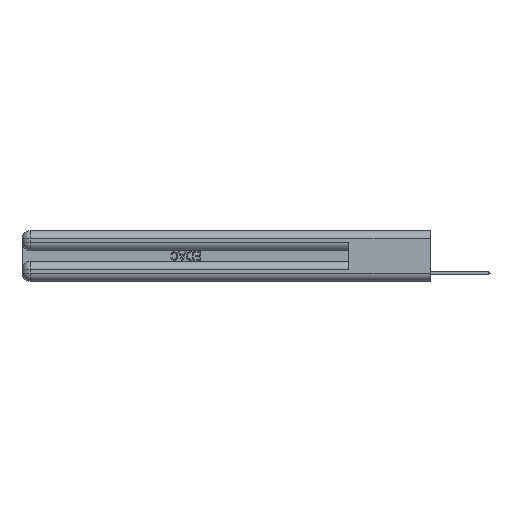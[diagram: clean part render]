
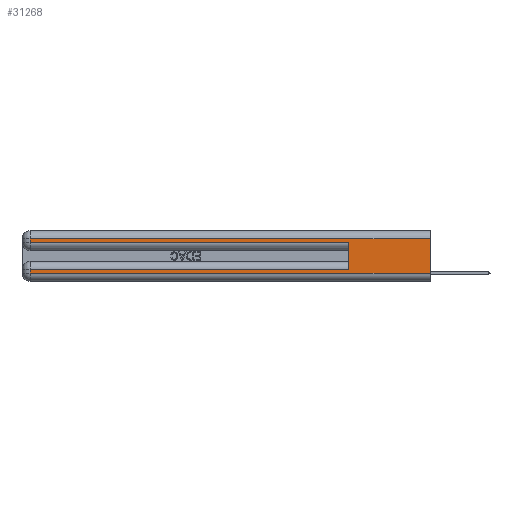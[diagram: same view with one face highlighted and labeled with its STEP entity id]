
A CAD part, left-side view. The second image highlights one B-rep face of the part: STEP entity #31268.
In plain terms, the highlighted planar face has unit normal (-1, 0, 0).
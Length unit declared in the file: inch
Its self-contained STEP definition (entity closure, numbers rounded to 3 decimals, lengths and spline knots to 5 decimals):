
#842 = DIRECTION ( 'NONE',  ( 0., 0., -1. ) ) ;
#1890 = LINE ( 'NONE', #7753, #27361 ) ;
#2162 = DIRECTION ( 'NONE',  ( 0., 0., -1. ) ) ;
#2788 = CARTESIAN_POINT ( 'NONE',  ( 0., 0., 0.085 ) ) ;
#2800 = VERTEX_POINT ( 'NONE', #10243 ) ;
#2830 = LINE ( 'NONE', #23119, #6940 ) ;
#3076 = VERTEX_POINT ( 'NONE', #11005 ) ;
#3846 = VERTEX_POINT ( 'NONE', #15947 ) ;
#3997 = CARTESIAN_POINT ( 'NONE',  ( 0., 2.94, 0.085 ) ) ;
#4005 = PLANE ( 'NONE',  #29487 ) ;
#4246 = VECTOR ( 'NONE', #32709, 39.37008 ) ;
#4670 = FACE_OUTER_BOUND ( 'NONE', #17009, .T. ) ;
#6491 = CARTESIAN_POINT ( 'NONE',  ( 0., 0.6, 0.145 ) ) ;
#6702 = VECTOR ( 'NONE', #842, 39.37008 ) ;
#6940 = VECTOR ( 'NONE', #13075, 39.37008 ) ;
#7240 = EDGE_CURVE ( 'NONE', #3846, #18724, #27258, .T. ) ;
#7455 = CARTESIAN_POINT ( 'NONE',  ( 0., 0., 0.37 ) ) ;
#7561 = LINE ( 'NONE', #21481, #6702 ) ;
#7753 = CARTESIAN_POINT ( 'NONE',  ( 0., 2.94, 0.37 ) ) ;
#7804 = DIRECTION ( 'NONE',  ( 0., 1., 0. ) ) ;
#8552 = EDGE_CURVE ( 'NONE', #9282, #28217, #1890, .T. ) ;
#9282 = VERTEX_POINT ( 'NONE', #3997 ) ;
#9346 = DIRECTION ( 'NONE',  ( 0., 0., 1. ) ) ;
#9461 = VERTEX_POINT ( 'NONE', #14901 ) ;
#10243 = CARTESIAN_POINT ( 'NONE',  ( 0., 0.6, 0.085 ) ) ;
#11005 = CARTESIAN_POINT ( 'NONE',  ( 0., 2.94, 0.285 ) ) ;
#11132 = EDGE_CURVE ( 'NONE', #2800, #9282, #13342, .T. ) ;
#12119 = ORIENTED_EDGE ( 'NONE', *, *, #7240, .F. ) ;
#12609 = LINE ( 'NONE', #17635, #4246 ) ;
#13075 = DIRECTION ( 'NONE',  ( 0., -1., 0. ) ) ;
#13342 = LINE ( 'NONE', #2788, #13940 ) ;
#13940 = VECTOR ( 'NONE', #7804, 39.37008 ) ;
#14241 = DIRECTION ( 'NONE',  ( 1., 0., 0. ) ) ;
#14245 = EDGE_CURVE ( 'NONE', #2800, #9461, #17071, .T. ) ;
#14858 = DIRECTION ( 'NONE',  ( 0., 0., -1. ) ) ;
#14901 = CARTESIAN_POINT ( 'NONE',  ( 0., 0.6, 0.285 ) ) ;
#14935 = CARTESIAN_POINT ( 'NONE',  ( 0., 0., 0.31 ) ) ;
#15297 = CARTESIAN_POINT ( 'NONE',  ( 0., 0., 0.06 ) ) ;
#15763 = CARTESIAN_POINT ( 'NONE',  ( 0., 2.94, 0.31 ) ) ;
#15947 = CARTESIAN_POINT ( 'NONE',  ( 0., 0., 0.31 ) ) ;
#17009 = EDGE_LOOP ( 'NONE', ( #12119, #31979, #25226, #32597, #28485, #19830, #26588, #25230 ) ) ;
#17071 = LINE ( 'NONE', #6491, #25682 ) ;
#17289 = DIRECTION ( 'NONE',  ( 0., 1., 0. ) ) ;
#17635 = CARTESIAN_POINT ( 'NONE',  ( 0., 0., 0.06 ) ) ;
#18127 = CARTESIAN_POINT ( 'NONE',  ( 0., 2.94, 0.06 ) ) ;
#18140 = VECTOR ( 'NONE', #17289, 39.37008 ) ;
#18724 = VERTEX_POINT ( 'NONE', #15297 ) ;
#19830 = ORIENTED_EDGE ( 'NONE', *, *, #11132, .T. ) ;
#20016 = DIRECTION ( 'NONE',  ( 0., 0., -1. ) ) ;
#21296 = EDGE_CURVE ( 'NONE', #21756, #3076, #7561, .T. ) ;
#21481 = CARTESIAN_POINT ( 'NONE',  ( 0., 2.94, 0.37 ) ) ;
#21756 = VERTEX_POINT ( 'NONE', #15763 ) ;
#23119 = CARTESIAN_POINT ( 'NONE',  ( 0., 0., 0.285 ) ) ;
#24799 = CARTESIAN_POINT ( 'NONE',  ( 0., 0., 0.37 ) ) ;
#24928 = EDGE_CURVE ( 'NONE', #3846, #21756, #27683, .T. ) ;
#25226 = ORIENTED_EDGE ( 'NONE', *, *, #21296, .T. ) ;
#25230 = ORIENTED_EDGE ( 'NONE', *, *, #28002, .T. ) ;
#25682 = VECTOR ( 'NONE', #9346, 39.37008 ) ;
#26588 = ORIENTED_EDGE ( 'NONE', *, *, #8552, .T. ) ;
#27258 = LINE ( 'NONE', #7455, #31748 ) ;
#27361 = VECTOR ( 'NONE', #20016, 39.37008 ) ;
#27683 = LINE ( 'NONE', #14935, #18140 ) ;
#28002 = EDGE_CURVE ( 'NONE', #28217, #18724, #12609, .T. ) ;
#28217 = VERTEX_POINT ( 'NONE', #18127 ) ;
#28485 = ORIENTED_EDGE ( 'NONE', *, *, #14245, .F. ) ;
#29487 = AXIS2_PLACEMENT_3D ( 'NONE', #24799, #14241, #2162 ) ;
#30270 = EDGE_CURVE ( 'NONE', #3076, #9461, #2830, .T. ) ;
#31268 = ADVANCED_FACE ( 'NONE', ( #4670 ), #4005, .F. ) ;
#31748 = VECTOR ( 'NONE', #14858, 39.37008 ) ;
#31979 = ORIENTED_EDGE ( 'NONE', *, *, #24928, .T. ) ;
#32597 = ORIENTED_EDGE ( 'NONE', *, *, #30270, .T. ) ;
#32709 = DIRECTION ( 'NONE',  ( 0., -1., 0. ) ) ;
